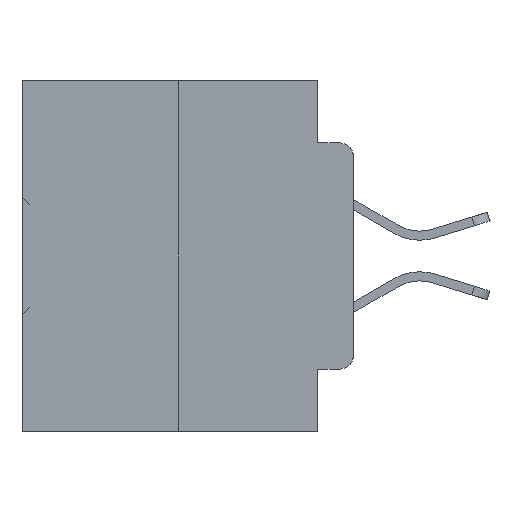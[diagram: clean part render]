
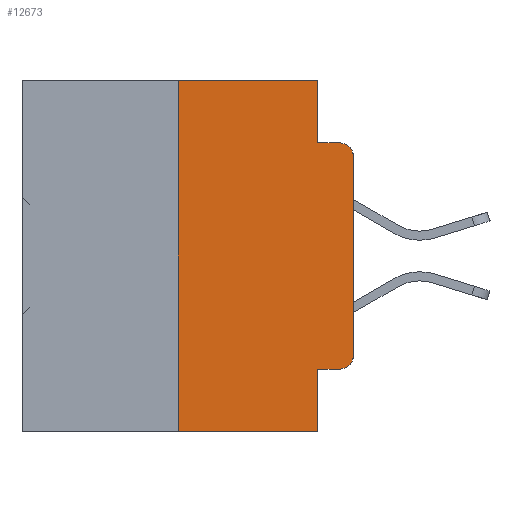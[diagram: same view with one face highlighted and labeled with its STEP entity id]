
A CAD part, left-side view. The second image highlights one B-rep face of the part: STEP entity #12673.
In plain terms, the highlighted planar face has unit normal (-1, 0, 0).
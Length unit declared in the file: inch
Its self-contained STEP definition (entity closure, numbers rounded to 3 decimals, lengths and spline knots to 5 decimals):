
#671 = LINE ( 'NONE', #11772, #12942 ) ;
#992 = DIRECTION ( 'NONE',  ( 1., 0., 0. ) ) ;
#1220 = CARTESIAN_POINT ( 'NONE',  ( 0., 0.02, -0.4115 ) ) ;
#1410 = VECTOR ( 'NONE', #28884, 39.37008 ) ;
#1520 = ORIENTED_EDGE ( 'NONE', *, *, #34270, .F. ) ;
#2787 = VECTOR ( 'NONE', #6989, 39.37008 ) ;
#3036 = DIRECTION ( 'NONE',  ( 0., 0., 1. ) ) ;
#4028 = CIRCLE ( 'NONE', #31417, 0.02 ) ;
#4876 = CARTESIAN_POINT ( 'NONE',  ( 0., 0.473, 0. ) ) ;
#5314 = VECTOR ( 'NONE', #37043, 39.37008 ) ;
#5336 = ORIENTED_EDGE ( 'NONE', *, *, #34734, .T. ) ;
#5752 = FACE_OUTER_BOUND ( 'NONE', #8451, .T. ) ;
#6467 = CARTESIAN_POINT ( 'NONE',  ( 0., 0.051, -0.0885 ) ) ;
#6575 = LINE ( 'NONE', #21095, #33959 ) ;
#6989 = DIRECTION ( 'NONE',  ( 0., 0., 1. ) ) ;
#7320 = CARTESIAN_POINT ( 'NONE',  ( 0., 0., -0.3915 ) ) ;
#8330 = CARTESIAN_POINT ( 'NONE',  ( 0., 0.051, 0. ) ) ;
#8386 = LINE ( 'NONE', #4876, #8827 ) ;
#8451 = EDGE_LOOP ( 'NONE', ( #19777, #27310, #28691, #26049, #1520, #18851, #27232, #21976, #5336, #22142 ) ) ;
#8827 = VECTOR ( 'NONE', #25958, 39.37008 ) ;
#8862 = DIRECTION ( 'NONE',  ( 0., -1., 0. ) ) ;
#8863 = VERTEX_POINT ( 'NONE', #32355 ) ;
#9779 = VECTOR ( 'NONE', #13822, 39.37008 ) ;
#9939 = LINE ( 'NONE', #33871, #5314 ) ;
#9953 = CARTESIAN_POINT ( 'NONE',  ( 0., 0.051, -0.4115 ) ) ;
#11375 = DIRECTION ( 'NONE',  ( 0., 0., -1. ) ) ;
#11438 = VERTEX_POINT ( 'NONE', #8330 ) ;
#11696 = CARTESIAN_POINT ( 'NONE',  ( 0., 0., -0.1085 ) ) ;
#11746 = LINE ( 'NONE', #16598, #9779 ) ;
#11772 = CARTESIAN_POINT ( 'NONE',  ( 0., 0.051, -0.0885 ) ) ;
#12147 = AXIS2_PLACEMENT_3D ( 'NONE', #17342, #20375, #11375 ) ;
#12591 = CIRCLE ( 'NONE', #12147, 0.02 ) ;
#12673 = ADVANCED_FACE ( 'NONE', ( #5752 ), #22317, .F. ) ;
#12942 = VECTOR ( 'NONE', #8862, 39.37008 ) ;
#13340 = CARTESIAN_POINT ( 'NONE',  ( 0., 0.25, 0. ) ) ;
#13822 = DIRECTION ( 'NONE',  ( 0., 0., -1. ) ) ;
#14447 = VERTEX_POINT ( 'NONE', #30984 ) ;
#16149 = CARTESIAN_POINT ( 'NONE',  ( 0., 0.051, -0.4115 ) ) ;
#16598 = CARTESIAN_POINT ( 'NONE',  ( 0., 0.051, 0. ) ) ;
#17006 = LINE ( 'NONE', #22571, #1410 ) ;
#17342 = CARTESIAN_POINT ( 'NONE',  ( 0., 0.02, -0.1085 ) ) ;
#17819 = EDGE_CURVE ( 'NONE', #19091, #14447, #9939, .T. ) ;
#18851 = ORIENTED_EDGE ( 'NONE', *, *, #32312, .F. ) ;
#19014 = CARTESIAN_POINT ( 'NONE',  ( 0., 0.473, 0. ) ) ;
#19091 = VERTEX_POINT ( 'NONE', #37816 ) ;
#19777 = ORIENTED_EDGE ( 'NONE', *, *, #38756, .T. ) ;
#19823 = EDGE_CURVE ( 'NONE', #27772, #38886, #12591, .T. ) ;
#20370 = VERTEX_POINT ( 'NONE', #6467 ) ;
#20375 = DIRECTION ( 'NONE',  ( -1., 0., 0. ) ) ;
#21095 = CARTESIAN_POINT ( 'NONE',  ( 0., 0., 0. ) ) ;
#21976 = ORIENTED_EDGE ( 'NONE', *, *, #31800, .F. ) ;
#22052 = DIRECTION ( 'NONE',  ( 0., 0., -1. ) ) ;
#22142 = ORIENTED_EDGE ( 'NONE', *, *, #22446, .T. ) ;
#22317 = PLANE ( 'NONE',  #33433 ) ;
#22446 = EDGE_CURVE ( 'NONE', #26002, #22492, #4028, .T. ) ;
#22492 = VERTEX_POINT ( 'NONE', #7320 ) ;
#22571 = CARTESIAN_POINT ( 'NONE',  ( 0., 0.051, 0. ) ) ;
#22655 = DIRECTION ( 'NONE',  ( -1., 0., 0. ) ) ;
#25958 = DIRECTION ( 'NONE',  ( 0., -1., 0. ) ) ;
#26002 = VERTEX_POINT ( 'NONE', #1220 ) ;
#26026 = EDGE_CURVE ( 'NONE', #11438, #20370, #17006, .T. ) ;
#26049 = ORIENTED_EDGE ( 'NONE', *, *, #26026, .F. ) ;
#27232 = ORIENTED_EDGE ( 'NONE', *, *, #17819, .T. ) ;
#27310 = ORIENTED_EDGE ( 'NONE', *, *, #19823, .T. ) ;
#27772 = VERTEX_POINT ( 'NONE', #11696 ) ;
#28138 = EDGE_CURVE ( 'NONE', #20370, #38886, #671, .T. ) ;
#28285 = CARTESIAN_POINT ( 'NONE',  ( 0., 0.02, -0.3915 ) ) ;
#28691 = ORIENTED_EDGE ( 'NONE', *, *, #28138, .F. ) ;
#28884 = DIRECTION ( 'NONE',  ( 0., 0., -1. ) ) ;
#30984 = CARTESIAN_POINT ( 'NONE',  ( 0., 0.051, -0.5 ) ) ;
#31274 = DIRECTION ( 'NONE',  ( 0., 0., -1. ) ) ;
#31417 = AXIS2_PLACEMENT_3D ( 'NONE', #28285, #22655, #31274 ) ;
#31800 = EDGE_CURVE ( 'NONE', #38344, #14447, #11746, .T. ) ;
#32312 = EDGE_CURVE ( 'NONE', #19091, #8863, #33364, .T. ) ;
#32355 = CARTESIAN_POINT ( 'NONE',  ( 0., 0.25, 0. ) ) ;
#33364 = LINE ( 'NONE', #13340, #2787 ) ;
#33433 = AXIS2_PLACEMENT_3D ( 'NONE', #19014, #992, #22052 ) ;
#33463 = CARTESIAN_POINT ( 'NONE',  ( 0., 0.02, -0.0885 ) ) ;
#33871 = CARTESIAN_POINT ( 'NONE',  ( 0., 0.473, -0.5 ) ) ;
#33926 = DIRECTION ( 'NONE',  ( 0., -1., 0. ) ) ;
#33959 = VECTOR ( 'NONE', #3036, 39.37008 ) ;
#34270 = EDGE_CURVE ( 'NONE', #8863, #11438, #8386, .T. ) ;
#34734 = EDGE_CURVE ( 'NONE', #38344, #26002, #36591, .T. ) ;
#35707 = VECTOR ( 'NONE', #33926, 39.37008 ) ;
#36591 = LINE ( 'NONE', #16149, #35707 ) ;
#37043 = DIRECTION ( 'NONE',  ( 0., -1., 0. ) ) ;
#37816 = CARTESIAN_POINT ( 'NONE',  ( 0., 0.25, -0.5 ) ) ;
#38344 = VERTEX_POINT ( 'NONE', #9953 ) ;
#38756 = EDGE_CURVE ( 'NONE', #22492, #27772, #6575, .T. ) ;
#38886 = VERTEX_POINT ( 'NONE', #33463 ) ;
